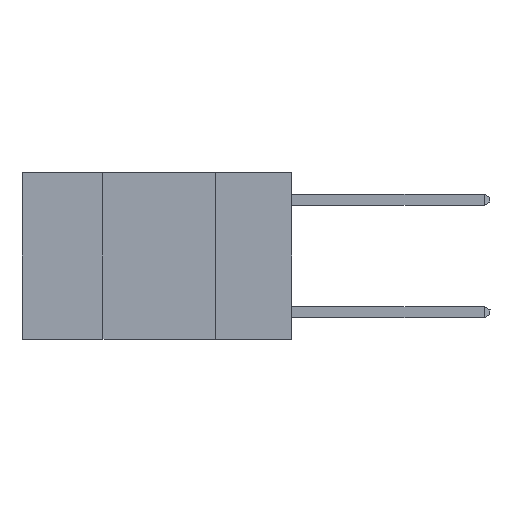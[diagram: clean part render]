
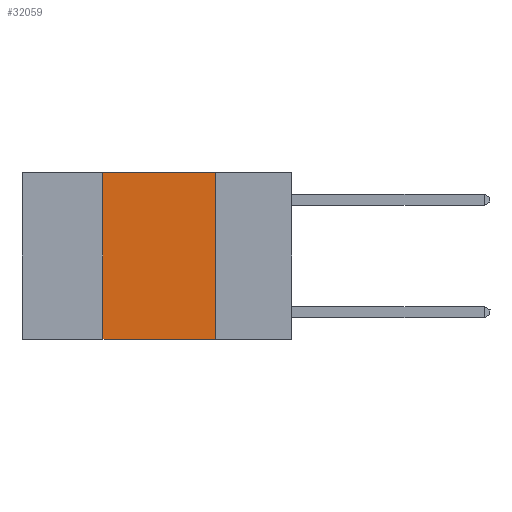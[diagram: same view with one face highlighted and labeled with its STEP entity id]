
A CAD part, left-side view. The second image highlights one B-rep face of the part: STEP entity #32059.
In plain terms, the highlighted planar face has unit normal (-1, 0, 0).
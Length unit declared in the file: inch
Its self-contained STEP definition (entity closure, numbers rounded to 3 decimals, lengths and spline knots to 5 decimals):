
#562 = VERTEX_POINT ( 'NONE', #32240 ) ;
#1273 = CARTESIAN_POINT ( 'NONE',  ( 0., 0.6, 0. ) ) ;
#2798 = LINE ( 'NONE', #15397, #22186 ) ;
#2971 = AXIS2_PLACEMENT_3D ( 'NONE', #32050, #7182, #24809 ) ;
#3462 = CARTESIAN_POINT ( 'NONE',  ( 0., 0.42, -0.37 ) ) ;
#4791 = LINE ( 'NONE', #14945, #24901 ) ;
#5457 = ORIENTED_EDGE ( 'NONE', *, *, #20214, .F. ) ;
#6507 = EDGE_CURVE ( 'NONE', #29474, #562, #2798, .T. ) ;
#7182 = DIRECTION ( 'NONE',  ( 1., 0., 0. ) ) ;
#7897 = DIRECTION ( 'NONE',  ( 0., 0., 1. ) ) ;
#8556 = EDGE_LOOP ( 'NONE', ( #24055, #5457, #16712, #20988 ) ) ;
#8575 = VECTOR ( 'NONE', #27607, 39.37008 ) ;
#9072 = CARTESIAN_POINT ( 'NONE',  ( 0., 0.17, -0.37 ) ) ;
#9641 = PLANE ( 'NONE',  #2971 ) ;
#10011 = DIRECTION ( 'NONE',  ( 0., 0., -1. ) ) ;
#10709 = EDGE_CURVE ( 'NONE', #25471, #11718, #4791, .T. ) ;
#11426 = DIRECTION ( 'NONE',  ( 0., -1., 0. ) ) ;
#11718 = VERTEX_POINT ( 'NONE', #9072 ) ;
#11970 = FACE_OUTER_BOUND ( 'NONE', #8556, .T. ) ;
#11995 = CARTESIAN_POINT ( 'NONE',  ( 0., 0.17, 0. ) ) ;
#14945 = CARTESIAN_POINT ( 'NONE',  ( 0., 0.17, 0. ) ) ;
#15397 = CARTESIAN_POINT ( 'NONE',  ( 0., 0.42, 0. ) ) ;
#16712 = ORIENTED_EDGE ( 'NONE', *, *, #6507, .F. ) ;
#16755 = VECTOR ( 'NONE', #11426, 39.37008 ) ;
#18473 = EDGE_CURVE ( 'NONE', #29474, #11718, #31614, .T. ) ;
#20090 = CARTESIAN_POINT ( 'NONE',  ( 0., 0.6, -0.37 ) ) ;
#20214 = EDGE_CURVE ( 'NONE', #562, #25471, #23451, .T. ) ;
#20988 = ORIENTED_EDGE ( 'NONE', *, *, #18473, .T. ) ;
#22186 = VECTOR ( 'NONE', #7897, 39.37008 ) ;
#23451 = LINE ( 'NONE', #1273, #16755 ) ;
#24055 = ORIENTED_EDGE ( 'NONE', *, *, #10709, .F. ) ;
#24809 = DIRECTION ( 'NONE',  ( 0., 0., -1. ) ) ;
#24901 = VECTOR ( 'NONE', #10011, 39.37008 ) ;
#25471 = VERTEX_POINT ( 'NONE', #11995 ) ;
#27607 = DIRECTION ( 'NONE',  ( 0., -1., 0. ) ) ;
#29474 = VERTEX_POINT ( 'NONE', #3462 ) ;
#31614 = LINE ( 'NONE', #20090, #8575 ) ;
#32050 = CARTESIAN_POINT ( 'NONE',  ( 0., 0.6, 0. ) ) ;
#32059 = ADVANCED_FACE ( 'NONE', ( #11970 ), #9641, .F. ) ;
#32240 = CARTESIAN_POINT ( 'NONE',  ( 0., 0.42, 0. ) ) ;
